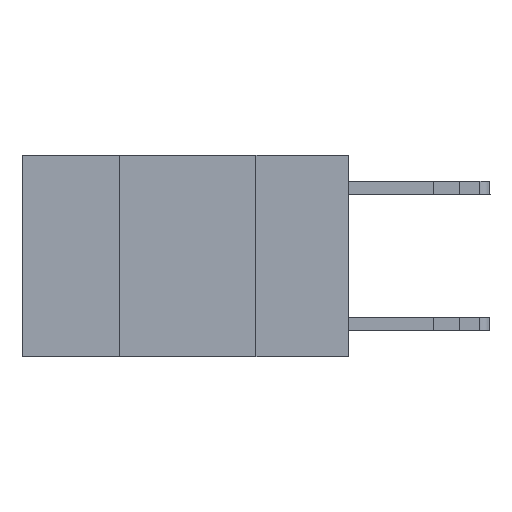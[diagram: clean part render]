
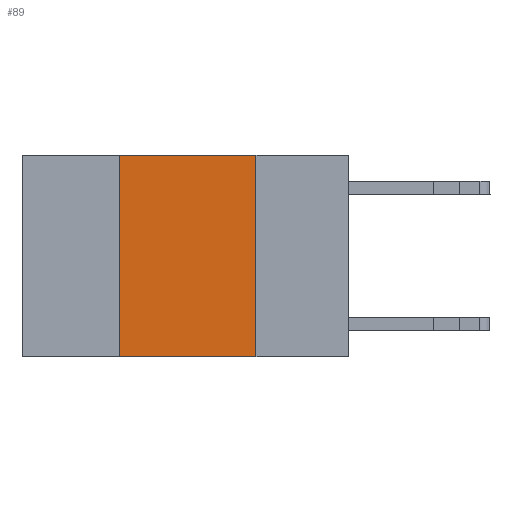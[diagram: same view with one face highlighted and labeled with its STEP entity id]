
A CAD part, left-side view. The second image highlights one B-rep face of the part: STEP entity #89.
In plain terms, the highlighted planar face has unit normal (-1, 0, 0).
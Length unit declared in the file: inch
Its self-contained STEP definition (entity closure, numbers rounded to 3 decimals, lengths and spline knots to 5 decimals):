
#54 = VERTEX_POINT ( 'NONE', #2969 ) ;
#89 = ADVANCED_FACE ( 'NONE', ( #12241 ), #5116, .F. ) ;
#595 = DIRECTION ( 'NONE',  ( 1., 0., 0. ) ) ;
#930 = VECTOR ( 'NONE', #11555, 39.37008 ) ;
#1181 = CARTESIAN_POINT ( 'NONE',  ( 0., 0.42, 0. ) ) ;
#1485 = ORIENTED_EDGE ( 'NONE', *, *, #4044, .F. ) ;
#1618 = ORIENTED_EDGE ( 'NONE', *, *, #7905, .F. ) ;
#1968 = CARTESIAN_POINT ( 'NONE',  ( 0., 0.6, 0. ) ) ;
#2253 = CARTESIAN_POINT ( 'NONE',  ( 0., 0.17, 0. ) ) ;
#2381 = ORIENTED_EDGE ( 'NONE', *, *, #6925, .F. ) ;
#2913 = LINE ( 'NONE', #7802, #11336 ) ;
#2969 = CARTESIAN_POINT ( 'NONE',  ( 0., 0.42, -0.37 ) ) ;
#3784 = EDGE_LOOP ( 'NONE', ( #1618, #2381, #1485, #13321 ) ) ;
#4044 = EDGE_CURVE ( 'NONE', #54, #13332, #7204, .T. ) ;
#4792 = VECTOR ( 'NONE', #9347, 39.37008 ) ;
#5105 = CARTESIAN_POINT ( 'NONE',  ( 0., 0.17, 0. ) ) ;
#5116 = PLANE ( 'NONE',  #7473 ) ;
#5612 = CARTESIAN_POINT ( 'NONE',  ( 0., 0.17, -0.37 ) ) ;
#5616 = CARTESIAN_POINT ( 'NONE',  ( 0., 0.42, 0. ) ) ;
#5840 = VECTOR ( 'NONE', #9603, 39.37008 ) ;
#6886 = LINE ( 'NONE', #1968, #930 ) ;
#6925 = EDGE_CURVE ( 'NONE', #13332, #9709, #6886, .T. ) ;
#7204 = LINE ( 'NONE', #1181, #5840 ) ;
#7473 = AXIS2_PLACEMENT_3D ( 'NONE', #13609, #595, #8799 ) ;
#7802 = CARTESIAN_POINT ( 'NONE',  ( 0., 0.6, -0.37 ) ) ;
#7905 = EDGE_CURVE ( 'NONE', #9709, #13988, #10427, .T. ) ;
#8799 = DIRECTION ( 'NONE',  ( 0., 0., -1. ) ) ;
#9347 = DIRECTION ( 'NONE',  ( 0., 0., -1. ) ) ;
#9603 = DIRECTION ( 'NONE',  ( 0., 0., 1. ) ) ;
#9709 = VERTEX_POINT ( 'NONE', #5105 ) ;
#10427 = LINE ( 'NONE', #2253, #4792 ) ;
#11336 = VECTOR ( 'NONE', #14733, 39.37008 ) ;
#11555 = DIRECTION ( 'NONE',  ( 0., -1., 0. ) ) ;
#12241 = FACE_OUTER_BOUND ( 'NONE', #3784, .T. ) ;
#13321 = ORIENTED_EDGE ( 'NONE', *, *, #13727, .T. ) ;
#13332 = VERTEX_POINT ( 'NONE', #5616 ) ;
#13609 = CARTESIAN_POINT ( 'NONE',  ( 0., 0.6, 0. ) ) ;
#13727 = EDGE_CURVE ( 'NONE', #54, #13988, #2913, .T. ) ;
#13988 = VERTEX_POINT ( 'NONE', #5612 ) ;
#14733 = DIRECTION ( 'NONE',  ( 0., -1., 0. ) ) ;
